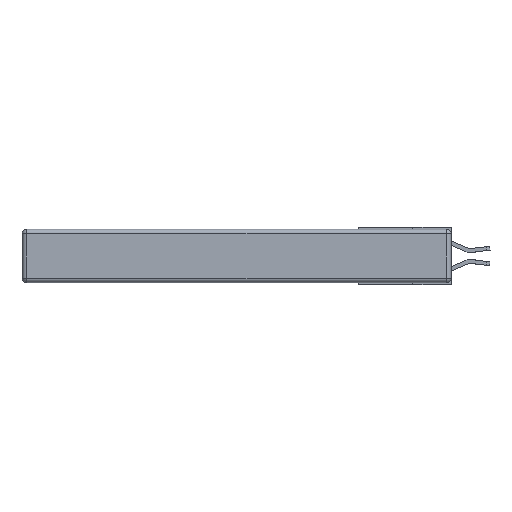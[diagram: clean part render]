
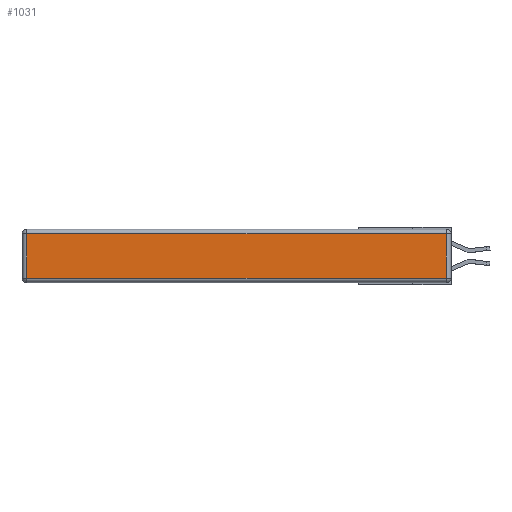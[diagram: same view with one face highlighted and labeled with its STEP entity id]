
A CAD part, left-side view. The second image highlights one B-rep face of the part: STEP entity #1031.
In plain terms, the highlighted planar face has unit normal (-1, 0, 0).
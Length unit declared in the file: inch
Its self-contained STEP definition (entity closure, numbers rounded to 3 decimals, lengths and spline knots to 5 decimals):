
#17 = FACE_OUTER_BOUND ( 'NONE', #796, .T. ) ;
#429 = DIRECTION ( 'NONE',  ( 0., 0., 1. ) ) ;
#524 = ORIENTED_EDGE ( 'NONE', *, *, #6557, .T. ) ;
#777 = CARTESIAN_POINT ( 'NONE',  ( 0., 2.72, -0.313 ) ) ;
#796 = EDGE_LOOP ( 'NONE', ( #12218, #524, #5852, #7616 ) ) ;
#829 = PLANE ( 'NONE',  #5003 ) ;
#879 = DIRECTION ( 'NONE',  ( 0., 0., 1. ) ) ;
#1031 = ADVANCED_FACE ( 'NONE', ( #17 ), #829, .T. ) ;
#1168 = VECTOR ( 'NONE', #2355, 39.37008 ) ;
#1227 = VECTOR ( 'NONE', #6343, 39.37008 ) ;
#1714 = VERTEX_POINT ( 'NONE', #9009 ) ;
#1800 = CARTESIAN_POINT ( 'NONE',  ( 0., 0., -0.343 ) ) ;
#2355 = DIRECTION ( 'NONE',  ( 0., 1., 0. ) ) ;
#2630 = LINE ( 'NONE', #5773, #4854 ) ;
#2649 = LINE ( 'NONE', #8110, #1168 ) ;
#3649 = DIRECTION ( 'NONE',  ( -1., 0., 0. ) ) ;
#3738 = LINE ( 'NONE', #11244, #1227 ) ;
#3924 = EDGE_CURVE ( 'NONE', #1714, #9255, #2649, .T. ) ;
#4010 = CARTESIAN_POINT ( 'NONE',  ( 0., 0.03, -0.313 ) ) ;
#4854 = VECTOR ( 'NONE', #429, 39.37008 ) ;
#5003 = AXIS2_PLACEMENT_3D ( 'NONE', #1800, #3649, #879 ) ;
#5083 = VERTEX_POINT ( 'NONE', #777 ) ;
#5773 = CARTESIAN_POINT ( 'NONE',  ( 0., 0.03, -0.343 ) ) ;
#5852 = ORIENTED_EDGE ( 'NONE', *, *, #3924, .T. ) ;
#6343 = DIRECTION ( 'NONE',  ( 0., -1., 0. ) ) ;
#6557 = EDGE_CURVE ( 'NONE', #7934, #1714, #2630, .T. ) ;
#6897 = DIRECTION ( 'NONE',  ( 0., 0., -1. ) ) ;
#7616 = ORIENTED_EDGE ( 'NONE', *, *, #7909, .T. ) ;
#7713 = CARTESIAN_POINT ( 'NONE',  ( 0., 2.72, -0.03 ) ) ;
#7830 = CARTESIAN_POINT ( 'NONE',  ( 0., 2.72, -0.343 ) ) ;
#7909 = EDGE_CURVE ( 'NONE', #9255, #5083, #12048, .T. ) ;
#7934 = VERTEX_POINT ( 'NONE', #4010 ) ;
#7987 = VECTOR ( 'NONE', #6897, 39.37008 ) ;
#8110 = CARTESIAN_POINT ( 'NONE',  ( 0., 2.75, -0.03 ) ) ;
#9009 = CARTESIAN_POINT ( 'NONE',  ( 0., 0.03, -0.03 ) ) ;
#9255 = VERTEX_POINT ( 'NONE', #7713 ) ;
#9584 = EDGE_CURVE ( 'NONE', #5083, #7934, #3738, .T. ) ;
#11244 = CARTESIAN_POINT ( 'NONE',  ( 0., 0., -0.313 ) ) ;
#12048 = LINE ( 'NONE', #7830, #7987 ) ;
#12218 = ORIENTED_EDGE ( 'NONE', *, *, #9584, .T. ) ;
